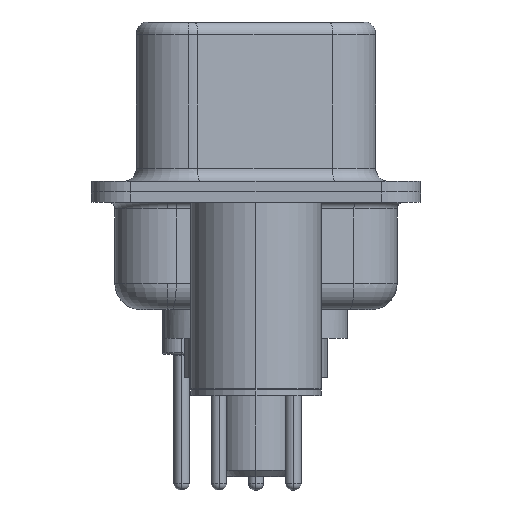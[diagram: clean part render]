
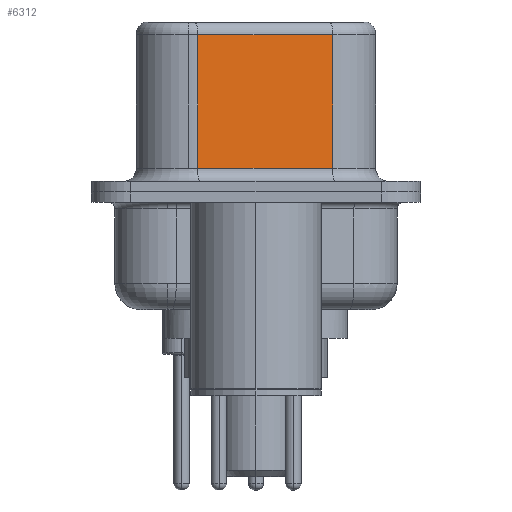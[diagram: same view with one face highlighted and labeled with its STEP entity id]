
A CAD part, left-side view. The second image highlights one B-rep face of the part: STEP entity #6312.
In plain terms, the highlighted planar face has unit normal (-0.985, -0.174, 0).
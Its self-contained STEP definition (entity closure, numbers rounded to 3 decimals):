
#57 = CARTESIAN_POINT ( 'NONE',  ( 4.585, -2.927, 6.52 ) ) ;
#202 = ORIENTED_EDGE ( 'NONE', *, *, #9206, .T. ) ;
#453 = CARTESIAN_POINT ( 'NONE',  ( 4.585, -2.927, 6.02 ) ) ;
#2129 = VERTEX_POINT ( 'NONE', #11456 ) ;
#2497 = EDGE_CURVE ( 'NONE', #14691, #21284, #9998, .T. ) ;
#2830 = ORIENTED_EDGE ( 'NONE', *, *, #2497, .T. ) ;
#3604 = ORIENTED_EDGE ( 'NONE', *, *, #23394, .F. ) ;
#3713 = VECTOR ( 'NONE', #19809, 1000. ) ;
#4247 = VERTEX_POINT ( 'NONE', #453 ) ;
#4893 = DIRECTION ( 'NONE',  ( 0., 0., -1. ) ) ;
#5910 = DIRECTION ( 'NONE',  ( -0.174, 0.985, 0. ) ) ;
#6312 = ADVANCED_FACE ( 'NONE', ( #6562 ), #23012, .F. ) ;
#6562 = FACE_OUTER_BOUND ( 'NONE', #16922, .T. ) ;
#7111 = LINE ( 'NONE', #18850, #21194 ) ;
#7161 = EDGE_CURVE ( 'NONE', #4247, #14691, #7111, .T. ) ;
#7429 = DIRECTION ( 'NONE',  ( 0., 0., -1. ) ) ;
#8278 = CARTESIAN_POINT ( 'NONE',  ( 3.675, 2.233, 6.02 ) ) ;
#9206 = EDGE_CURVE ( 'NONE', #21284, #2129, #11208, .T. ) ;
#9305 = ORIENTED_EDGE ( 'NONE', *, *, #7161, .T. ) ;
#9998 = LINE ( 'NONE', #19982, #22048 ) ;
#11208 = LINE ( 'NONE', #15967, #3713 ) ;
#11456 = CARTESIAN_POINT ( 'NONE',  ( 4.585, -2.927, 0.9 ) ) ;
#11682 = DIRECTION ( 'NONE',  ( 0.985, 0.174, 0. ) ) ;
#12348 = AXIS2_PLACEMENT_3D ( 'NONE', #57, #11682, #5910 ) ;
#13396 = DIRECTION ( 'NONE',  ( -0.174, 0.985, 0. ) ) ;
#14098 = LINE ( 'NONE', #18749, #24603 ) ;
#14691 = VERTEX_POINT ( 'NONE', #8278 ) ;
#15967 = CARTESIAN_POINT ( 'NONE',  ( 4.585, -2.927, 0.9 ) ) ;
#16922 = EDGE_LOOP ( 'NONE', ( #3604, #9305, #2830, #202 ) ) ;
#18749 = CARTESIAN_POINT ( 'NONE',  ( 4.585, -2.927, 6.52 ) ) ;
#18850 = CARTESIAN_POINT ( 'NONE',  ( 4.585, -2.927, 6.02 ) ) ;
#19809 = DIRECTION ( 'NONE',  ( 0.174, -0.985, 0. ) ) ;
#19885 = CARTESIAN_POINT ( 'NONE',  ( 3.675, 2.233, 0.9 ) ) ;
#19982 = CARTESIAN_POINT ( 'NONE',  ( 3.675, 2.233, 6.52 ) ) ;
#21194 = VECTOR ( 'NONE', #13396, 1000. ) ;
#21284 = VERTEX_POINT ( 'NONE', #19885 ) ;
#22048 = VECTOR ( 'NONE', #4893, 1000. ) ;
#23012 = PLANE ( 'NONE',  #12348 ) ;
#23394 = EDGE_CURVE ( 'NONE', #4247, #2129, #14098, .T. ) ;
#24603 = VECTOR ( 'NONE', #7429, 1000. ) ;
